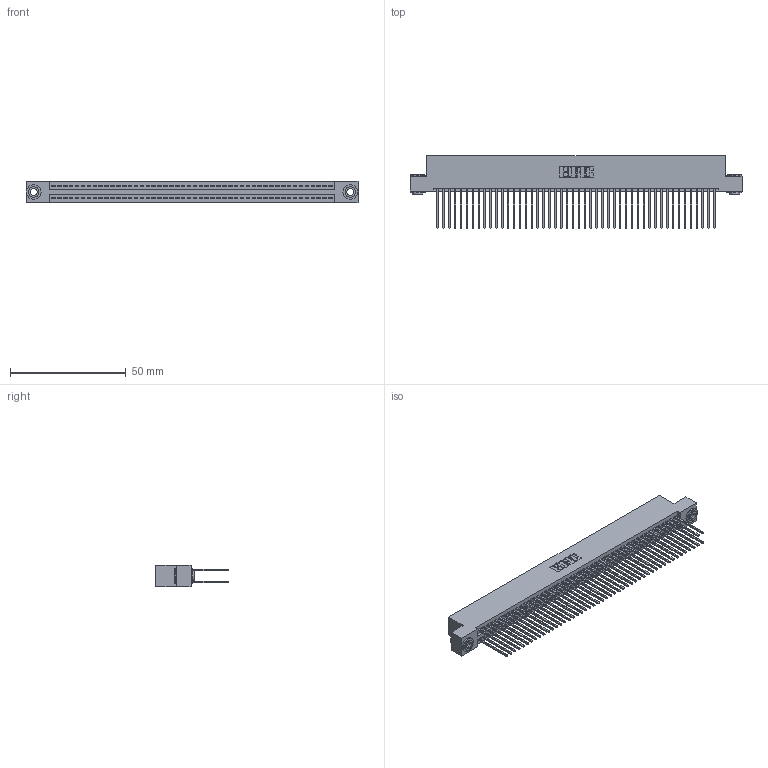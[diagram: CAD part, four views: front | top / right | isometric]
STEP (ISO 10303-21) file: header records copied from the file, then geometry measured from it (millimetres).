
FILE_DESCRIPTION (( 'STEP AP203' ), '1' );
FILE_NAME ('395-096-542-203.STEP', '2018-11-29T16:03:42', ( '' ), ( '' ), 'SwSTEP 2.0', 'SolidWorks 2016', '' );
FILE_SCHEMA (( 'CONFIG_CONTROL_DESIGN' ));
Length unit declared in the file: inch
Products named in the file (4): 345 Part_Flush Mounting Lugs - 0.156 Dia-TH; 395-096-542-203; 345-250-002_345-250-002-102; 345-292-001_345-293-142
Assembly tree (99 placements, depth 2):
  395-096-542-203
    345 Part_Flush Mounting Lugs - 0.156 Dia-TH
    345-292-001_345-293-142  x96
    345-250-002_345-250-002-102  x2
Bounding box: 143.13 x 31.29 x 9.4 mm (x, y, z)
Volume: 14426.3 mm3; surface area: 23736.9 mm2
Topology: 99 solids, 99 shells, 4964 faces, 14721 edges, 9682 vertices
Faces by surface type: plane 3258, cylinder 1698, cone 8
Entity records: 37522 total; most frequent: CARTESIAN_POINT 6259, ORIENTED_EDGE 6186, DIRECTION 5543, EDGE_CURVE 3093, VECTOR 2745, LINE 2745, VERTEX_POINT 2058, AXIS2_PLACEMENT_3D 1399
